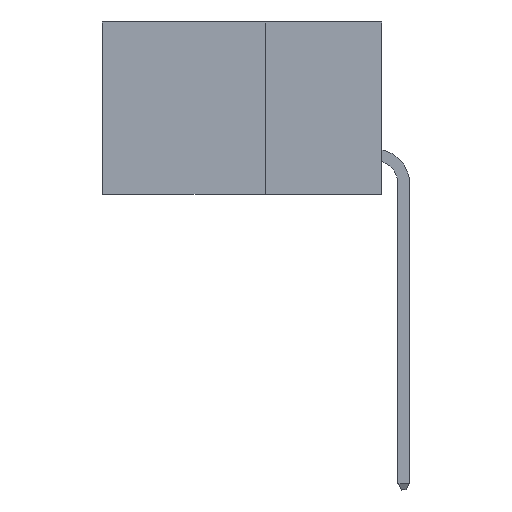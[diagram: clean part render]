
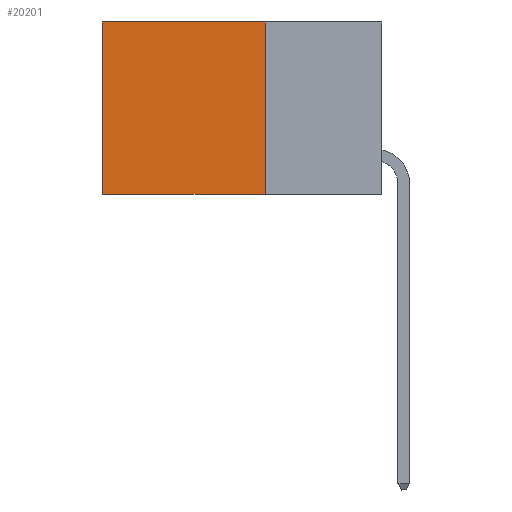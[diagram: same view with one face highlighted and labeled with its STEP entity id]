
A CAD part, left-side view. The second image highlights one B-rep face of the part: STEP entity #20201.
In plain terms, the highlighted planar face has unit normal (-1, 0, 0).
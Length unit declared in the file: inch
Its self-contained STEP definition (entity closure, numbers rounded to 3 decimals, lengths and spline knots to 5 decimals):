
#690 = VECTOR ( 'NONE', #1561, 39.37008 ) ;
#914 = EDGE_CURVE ( 'NONE', #2696, #2385, #17030, .T. ) ;
#1484 = CARTESIAN_POINT ( 'NONE',  ( 0.2875, 0.25, 0. ) ) ;
#1561 = DIRECTION ( 'NONE',  ( 0., 1., 0. ) ) ;
#2270 = VECTOR ( 'NONE', #10290, 39.37008 ) ;
#2385 = VERTEX_POINT ( 'NONE', #14411 ) ;
#2696 = VERTEX_POINT ( 'NONE', #10534 ) ;
#2767 = LINE ( 'NONE', #3900, #2270 ) ;
#2907 = CARTESIAN_POINT ( 'NONE',  ( 0.2875, 0.25, 0. ) ) ;
#2927 = LINE ( 'NONE', #18837, #690 ) ;
#3121 = CARTESIAN_POINT ( 'NONE',  ( 0.2875, 0.6, 0. ) ) ;
#3900 = CARTESIAN_POINT ( 'NONE',  ( 0.2875, 0.25, 0. ) ) ;
#6875 = FACE_OUTER_BOUND ( 'NONE', #12892, .T. ) ;
#8254 = ORIENTED_EDGE ( 'NONE', *, *, #16829, .F. ) ;
#8528 = VERTEX_POINT ( 'NONE', #15181 ) ;
#9095 = DIRECTION ( 'NONE',  ( 0., 0., -1. ) ) ;
#9488 = VECTOR ( 'NONE', #9095, 39.37008 ) ;
#9711 = ORIENTED_EDGE ( 'NONE', *, *, #14796, .F. ) ;
#10290 = DIRECTION ( 'NONE',  ( 0., 1., 0. ) ) ;
#10534 = CARTESIAN_POINT ( 'NONE',  ( 0.2875, 0.6, 0. ) ) ;
#10603 = VERTEX_POINT ( 'NONE', #18541 ) ;
#12892 = EDGE_LOOP ( 'NONE', ( #15652, #9711, #8254, #16960 ) ) ;
#13361 = EDGE_CURVE ( 'NONE', #10603, #2696, #2767, .T. ) ;
#13746 = LINE ( 'NONE', #2907, #9488 ) ;
#14411 = CARTESIAN_POINT ( 'NONE',  ( 0.2875, 0.6, -0.37 ) ) ;
#14796 = EDGE_CURVE ( 'NONE', #8528, #2385, #2927, .T. ) ;
#15181 = CARTESIAN_POINT ( 'NONE',  ( 0.2875, 0.25, -0.37 ) ) ;
#15614 = PLANE ( 'NONE',  #17505 ) ;
#15652 = ORIENTED_EDGE ( 'NONE', *, *, #914, .T. ) ;
#15752 = DIRECTION ( 'NONE',  ( 1., 0., 0. ) ) ;
#15823 = DIRECTION ( 'NONE',  ( 0., 0., -1. ) ) ;
#16829 = EDGE_CURVE ( 'NONE', #10603, #8528, #13746, .T. ) ;
#16960 = ORIENTED_EDGE ( 'NONE', *, *, #13361, .T. ) ;
#17030 = LINE ( 'NONE', #3121, #17282 ) ;
#17282 = VECTOR ( 'NONE', #20401, 39.37008 ) ;
#17505 = AXIS2_PLACEMENT_3D ( 'NONE', #1484, #15752, #15823 ) ;
#18541 = CARTESIAN_POINT ( 'NONE',  ( 0.2875, 0.25, 0. ) ) ;
#18837 = CARTESIAN_POINT ( 'NONE',  ( 0.2875, 0.25, -0.37 ) ) ;
#20201 = ADVANCED_FACE ( 'NONE', ( #6875 ), #15614, .F. ) ;
#20401 = DIRECTION ( 'NONE',  ( 0., 0., -1. ) ) ;
